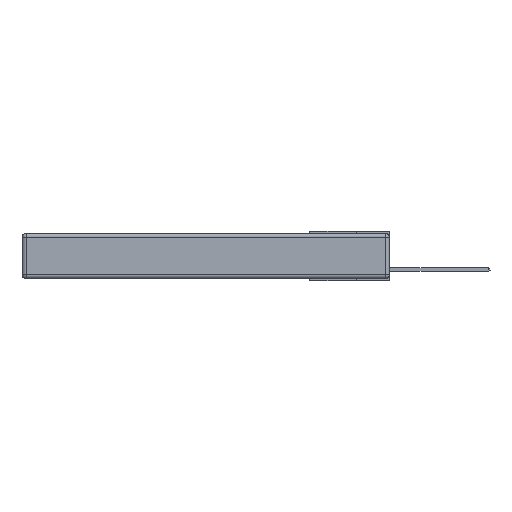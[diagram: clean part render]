
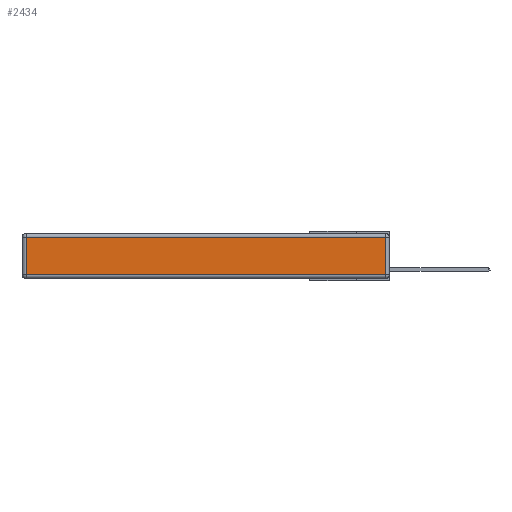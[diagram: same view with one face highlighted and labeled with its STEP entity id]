
A CAD part, left-side view. The second image highlights one B-rep face of the part: STEP entity #2434.
In plain terms, the highlighted planar face has unit normal (-1, 0, 0).
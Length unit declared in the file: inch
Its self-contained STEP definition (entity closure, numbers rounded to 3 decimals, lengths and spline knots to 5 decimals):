
#782 = CARTESIAN_POINT ( 'NONE',  ( 0., 0.03, -0.343 ) ) ;
#2128 = FACE_OUTER_BOUND ( 'NONE', #8263, .T. ) ;
#2396 = VECTOR ( 'NONE', #19598, 39.37008 ) ;
#2434 = ADVANCED_FACE ( 'NONE', ( #2128 ), #12314, .T. ) ;
#4379 = VECTOR ( 'NONE', #7544, 39.37008 ) ;
#4885 = ORIENTED_EDGE ( 'NONE', *, *, #6334, .T. ) ;
#6276 = VERTEX_POINT ( 'NONE', #24897 ) ;
#6334 = EDGE_CURVE ( 'NONE', #10735, #6276, #17782, .T. ) ;
#6795 = CARTESIAN_POINT ( 'NONE',  ( 0., 2.72, -0.313 ) ) ;
#7382 = ORIENTED_EDGE ( 'NONE', *, *, #15845, .T. ) ;
#7544 = DIRECTION ( 'NONE',  ( 0., 0., -1. ) ) ;
#7681 = LINE ( 'NONE', #22165, #10115 ) ;
#8263 = EDGE_LOOP ( 'NONE', ( #19001, #4885, #7382, #20909 ) ) ;
#10115 = VECTOR ( 'NONE', #20149, 39.37008 ) ;
#10735 = VERTEX_POINT ( 'NONE', #18686 ) ;
#11025 = LINE ( 'NONE', #16386, #4379 ) ;
#12119 = VECTOR ( 'NONE', #25761, 39.37008 ) ;
#12314 = PLANE ( 'NONE',  #18268 ) ;
#15845 = EDGE_CURVE ( 'NONE', #6276, #21014, #18203, .T. ) ;
#16386 = CARTESIAN_POINT ( 'NONE',  ( 0., 2.72, -0.343 ) ) ;
#17737 = EDGE_CURVE ( 'NONE', #24606, #10735, #7681, .T. ) ;
#17782 = LINE ( 'NONE', #782, #12119 ) ;
#18203 = LINE ( 'NONE', #25356, #2396 ) ;
#18268 = AXIS2_PLACEMENT_3D ( 'NONE', #21090, #28043, #27762 ) ;
#18686 = CARTESIAN_POINT ( 'NONE',  ( 0., 0.03, -0.313 ) ) ;
#19001 = ORIENTED_EDGE ( 'NONE', *, *, #17737, .T. ) ;
#19598 = DIRECTION ( 'NONE',  ( 0., 1., 0. ) ) ;
#20149 = DIRECTION ( 'NONE',  ( 0., -1., 0. ) ) ;
#20909 = ORIENTED_EDGE ( 'NONE', *, *, #28895, .T. ) ;
#21014 = VERTEX_POINT ( 'NONE', #25619 ) ;
#21090 = CARTESIAN_POINT ( 'NONE',  ( 0., 0., -0.343 ) ) ;
#22165 = CARTESIAN_POINT ( 'NONE',  ( 0., 0., -0.313 ) ) ;
#24606 = VERTEX_POINT ( 'NONE', #6795 ) ;
#24897 = CARTESIAN_POINT ( 'NONE',  ( 0., 0.03, -0.03 ) ) ;
#25356 = CARTESIAN_POINT ( 'NONE',  ( 0., 2.75, -0.03 ) ) ;
#25619 = CARTESIAN_POINT ( 'NONE',  ( 0., 2.72, -0.03 ) ) ;
#25761 = DIRECTION ( 'NONE',  ( 0., 0., 1. ) ) ;
#27762 = DIRECTION ( 'NONE',  ( 0., 0., 1. ) ) ;
#28043 = DIRECTION ( 'NONE',  ( -1., 0., 0. ) ) ;
#28895 = EDGE_CURVE ( 'NONE', #21014, #24606, #11025, .T. ) ;
